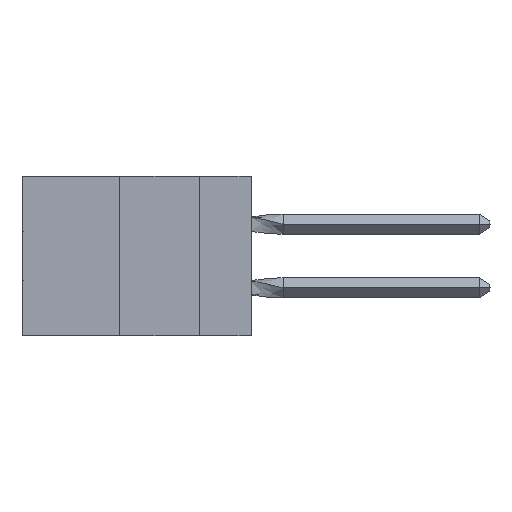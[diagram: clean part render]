
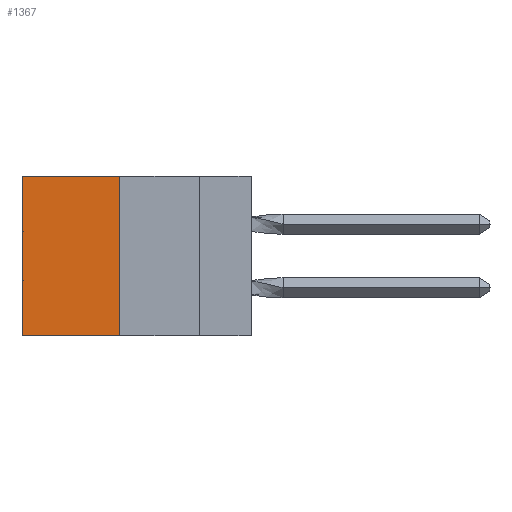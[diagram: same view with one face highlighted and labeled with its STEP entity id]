
A CAD part, left-side view. The second image highlights one B-rep face of the part: STEP entity #1367.
In plain terms, the highlighted planar face has unit normal (-1, 0, 0).
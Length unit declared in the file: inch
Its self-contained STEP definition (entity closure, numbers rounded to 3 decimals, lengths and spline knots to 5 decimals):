
#763 = DIRECTION ( 'NONE',  ( 0., 1., 0. ) ) ;
#1165 = EDGE_CURVE ( 'NONE', #33798, #28800, #26807, .T. ) ;
#1329 = CARTESIAN_POINT ( 'NONE',  ( 0.305, 0.72, -0.5 ) ) ;
#1367 = ADVANCED_FACE ( 'NONE', ( #22455 ), #19138, .F. ) ;
#4389 = VECTOR ( 'NONE', #17918, 39.37008 ) ;
#5219 = CARTESIAN_POINT ( 'NONE',  ( 0.305, 0.413, -0.5 ) ) ;
#5751 = VECTOR ( 'NONE', #763, 39.37008 ) ;
#5769 = EDGE_CURVE ( 'NONE', #33798, #14575, #10961, .T. ) ;
#6323 = VERTEX_POINT ( 'NONE', #1329 ) ;
#8685 = LINE ( 'NONE', #40942, #29409 ) ;
#9749 = AXIS2_PLACEMENT_3D ( 'NONE', #5219, #39631, #36262 ) ;
#10919 = EDGE_CURVE ( 'NONE', #28800, #6323, #28659, .T. ) ;
#10961 = LINE ( 'NONE', #15052, #4389 ) ;
#13429 = ORIENTED_EDGE ( 'NONE', *, *, #1165, .F. ) ;
#14575 = VERTEX_POINT ( 'NONE', #30534 ) ;
#15052 = CARTESIAN_POINT ( 'NONE',  ( 0.305, 0.413, 0. ) ) ;
#17918 = DIRECTION ( 'NONE',  ( 0., 1., 0. ) ) ;
#19138 = PLANE ( 'NONE',  #9749 ) ;
#22455 = FACE_OUTER_BOUND ( 'NONE', #34969, .T. ) ;
#26807 = LINE ( 'NONE', #34467, #33984 ) ;
#28659 = LINE ( 'NONE', #42481, #5751 ) ;
#28800 = VERTEX_POINT ( 'NONE', #45203 ) ;
#29409 = VECTOR ( 'NONE', #40642, 39.37008 ) ;
#30534 = CARTESIAN_POINT ( 'NONE',  ( 0.305, 0.72, 0. ) ) ;
#31070 = DIRECTION ( 'NONE',  ( 0., 0., -1. ) ) ;
#33798 = VERTEX_POINT ( 'NONE', #41637 ) ;
#33984 = VECTOR ( 'NONE', #31070, 39.37008 ) ;
#34467 = CARTESIAN_POINT ( 'NONE',  ( 0.305, 0.413, -0.5 ) ) ;
#34969 = EDGE_LOOP ( 'NONE', ( #39283, #38756, #13429, #40532 ) ) ;
#36262 = DIRECTION ( 'NONE',  ( 0., 0., -1. ) ) ;
#38756 = ORIENTED_EDGE ( 'NONE', *, *, #10919, .F. ) ;
#39283 = ORIENTED_EDGE ( 'NONE', *, *, #41612, .T. ) ;
#39631 = DIRECTION ( 'NONE',  ( 1., 0., 0. ) ) ;
#40532 = ORIENTED_EDGE ( 'NONE', *, *, #5769, .T. ) ;
#40642 = DIRECTION ( 'NONE',  ( 0., 0., -1. ) ) ;
#40942 = CARTESIAN_POINT ( 'NONE',  ( 0.305, 0.72, -0.5 ) ) ;
#41612 = EDGE_CURVE ( 'NONE', #14575, #6323, #8685, .T. ) ;
#41637 = CARTESIAN_POINT ( 'NONE',  ( 0.305, 0.413, 0. ) ) ;
#42481 = CARTESIAN_POINT ( 'NONE',  ( 0.305, 0.413, -0.5 ) ) ;
#45203 = CARTESIAN_POINT ( 'NONE',  ( 0.305, 0.413, -0.5 ) ) ;
